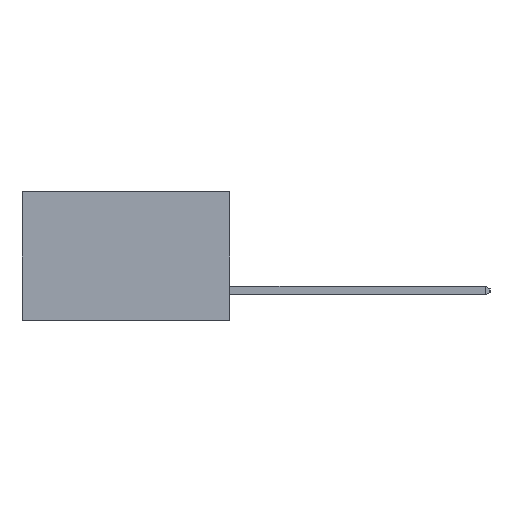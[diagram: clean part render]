
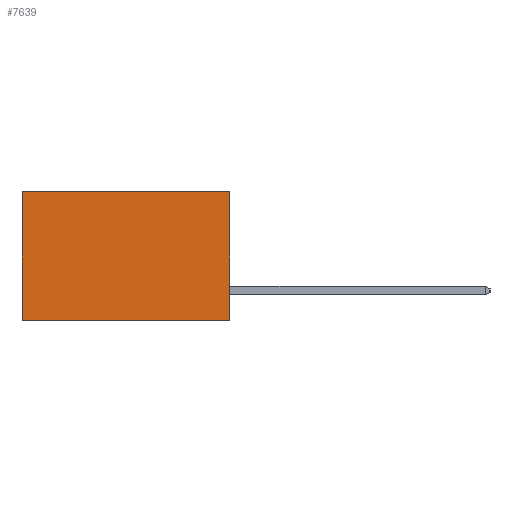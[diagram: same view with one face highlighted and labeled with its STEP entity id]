
A CAD part, left-side view. The second image highlights one B-rep face of the part: STEP entity #7639.
In plain terms, the highlighted planar face has unit normal (-1, 0, 0).
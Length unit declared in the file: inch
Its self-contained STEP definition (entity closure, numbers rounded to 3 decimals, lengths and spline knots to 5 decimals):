
#370 = VECTOR ( 'NONE', #7249, 39.37008 ) ;
#825 = CARTESIAN_POINT ( 'NONE',  ( 0.2615, 0.6, 0. ) ) ;
#873 = CARTESIAN_POINT ( 'NONE',  ( 0.2615, 0.6, -0.37 ) ) ;
#1027 = VECTOR ( 'NONE', #18636, 39.37008 ) ;
#2145 = LINE ( 'NONE', #873, #18080 ) ;
#2327 = CARTESIAN_POINT ( 'NONE',  ( 0.2615, 0., -0.37 ) ) ;
#2939 = ORIENTED_EDGE ( 'NONE', *, *, #12680, .F. ) ;
#3329 = FACE_OUTER_BOUND ( 'NONE', #17231, .T. ) ;
#3332 = ORIENTED_EDGE ( 'NONE', *, *, #16374, .T. ) ;
#4515 = CARTESIAN_POINT ( 'NONE',  ( 0.2615, 0., 0. ) ) ;
#6460 = AXIS2_PLACEMENT_3D ( 'NONE', #10177, #9816, #9798 ) ;
#7249 = DIRECTION ( 'NONE',  ( 0., 1., 0. ) ) ;
#7639 = ADVANCED_FACE ( 'NONE', ( #3329 ), #9864, .F. ) ;
#8452 = LINE ( 'NONE', #10501, #370 ) ;
#9798 = DIRECTION ( 'NONE',  ( 0., 0., -1. ) ) ;
#9816 = DIRECTION ( 'NONE',  ( 1., 0., 0. ) ) ;
#9864 = PLANE ( 'NONE',  #6460 ) ;
#10177 = CARTESIAN_POINT ( 'NONE',  ( 0.2615, 0., -0.37 ) ) ;
#10182 = LINE ( 'NONE', #2327, #1027 ) ;
#10501 = CARTESIAN_POINT ( 'NONE',  ( 0.2615, 0., 0. ) ) ;
#12680 = EDGE_CURVE ( 'NONE', #15390, #16233, #10182, .T. ) ;
#13205 = ORIENTED_EDGE ( 'NONE', *, *, #13848, .F. ) ;
#13429 = CARTESIAN_POINT ( 'NONE',  ( 0.2615, 0., -0.37 ) ) ;
#13848 = EDGE_CURVE ( 'NONE', #16233, #15768, #19319, .T. ) ;
#15048 = CARTESIAN_POINT ( 'NONE',  ( 0.2615, 0.6, -0.37 ) ) ;
#15294 = DIRECTION ( 'NONE',  ( 0., 0., -1. ) ) ;
#15390 = VERTEX_POINT ( 'NONE', #4515 ) ;
#15768 = VERTEX_POINT ( 'NONE', #15048 ) ;
#16034 = DIRECTION ( 'NONE',  ( 0., 1., 0. ) ) ;
#16079 = CARTESIAN_POINT ( 'NONE',  ( 0.2615, 0., -0.37 ) ) ;
#16233 = VERTEX_POINT ( 'NONE', #13429 ) ;
#16374 = EDGE_CURVE ( 'NONE', #17721, #15768, #2145, .T. ) ;
#17231 = EDGE_LOOP ( 'NONE', ( #3332, #13205, #2939, #20397 ) ) ;
#17721 = VERTEX_POINT ( 'NONE', #825 ) ;
#18080 = VECTOR ( 'NONE', #15294, 39.37008 ) ;
#18636 = DIRECTION ( 'NONE',  ( 0., 0., -1. ) ) ;
#18856 = VECTOR ( 'NONE', #16034, 39.37008 ) ;
#19319 = LINE ( 'NONE', #16079, #18856 ) ;
#19928 = EDGE_CURVE ( 'NONE', #15390, #17721, #8452, .T. ) ;
#20397 = ORIENTED_EDGE ( 'NONE', *, *, #19928, .T. ) ;
